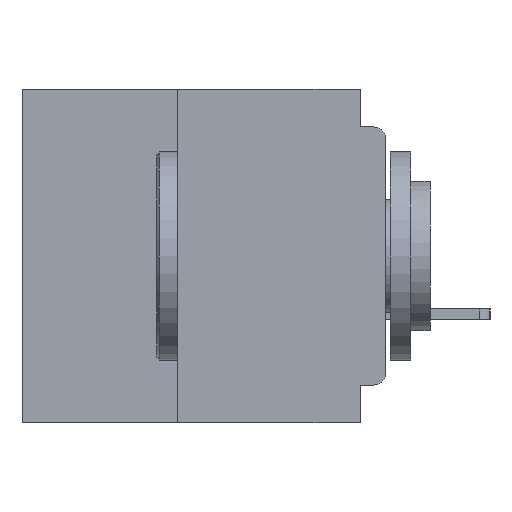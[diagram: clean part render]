
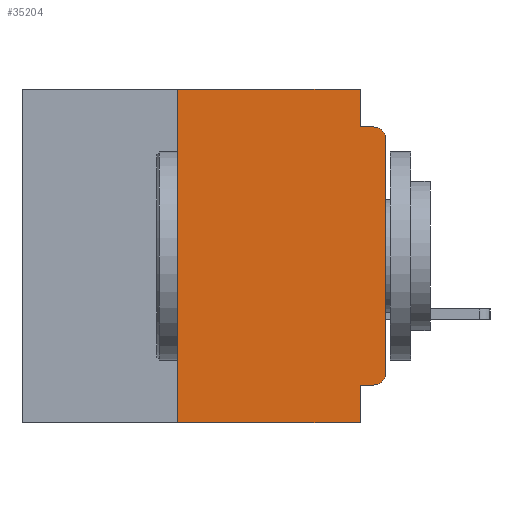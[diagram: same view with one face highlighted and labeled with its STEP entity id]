
A CAD part, left-side view. The second image highlights one B-rep face of the part: STEP entity #35204.
In plain terms, the highlighted planar face has unit normal (-1, 0, 0).
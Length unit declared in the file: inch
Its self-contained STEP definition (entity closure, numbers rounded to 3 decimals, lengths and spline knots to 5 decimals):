
#501 = DIRECTION ( 'NONE',  ( 0., -1., 0. ) ) ;
#698 = CARTESIAN_POINT ( 'NONE',  ( 0., 0.031, 0. ) ) ;
#894 = VECTOR ( 'NONE', #30926, 39.37008 ) ;
#3254 = CARTESIAN_POINT ( 'NONE',  ( 0., 0.25, -0.4 ) ) ;
#5697 = DIRECTION ( 'NONE',  ( 0., 0., -1. ) ) ;
#5958 = DIRECTION ( 'NONE',  ( -1., 0., 0. ) ) ;
#6098 = VERTEX_POINT ( 'NONE', #42554 ) ;
#6409 = CARTESIAN_POINT ( 'NONE',  ( 0., 0.015, -0.06 ) ) ;
#6439 = EDGE_CURVE ( 'NONE', #19492, #18868, #34185, .T. ) ;
#7051 = CARTESIAN_POINT ( 'NONE',  ( 0., 0., 0. ) ) ;
#7656 = LINE ( 'NONE', #34507, #42823 ) ;
#8656 = ORIENTED_EDGE ( 'NONE', *, *, #17409, .T. ) ;
#8794 = FACE_OUTER_BOUND ( 'NONE', #38263, .T. ) ;
#8994 = DIRECTION ( 'NONE',  ( 0., 0., 1. ) ) ;
#9819 = DIRECTION ( 'NONE',  ( 0., 0., -1. ) ) ;
#9920 = CARTESIAN_POINT ( 'NONE',  ( 0., 0., -0.34 ) ) ;
#10199 = EDGE_CURVE ( 'NONE', #22359, #40887, #28156, .T. ) ;
#10862 = LINE ( 'NONE', #26138, #29012 ) ;
#12484 = EDGE_CURVE ( 'NONE', #38335, #40887, #30149, .T. ) ;
#12596 = ORIENTED_EDGE ( 'NONE', *, *, #32562, .T. ) ;
#12644 = AXIS2_PLACEMENT_3D ( 'NONE', #14131, #17571, #41356 ) ;
#13024 = ORIENTED_EDGE ( 'NONE', *, *, #28829, .T. ) ;
#13084 = CARTESIAN_POINT ( 'NONE',  ( 0., 0.031, -0.355 ) ) ;
#14093 = DIRECTION ( 'NONE',  ( 0., 1., 0. ) ) ;
#14131 = CARTESIAN_POINT ( 'NONE',  ( 0., 0.437, 0. ) ) ;
#14196 = ORIENTED_EDGE ( 'NONE', *, *, #10199, .F. ) ;
#14395 = CIRCLE ( 'NONE', #21975, 0.015 ) ;
#16547 = EDGE_CURVE ( 'NONE', #18846, #35949, #22471, .T. ) ;
#17409 = EDGE_CURVE ( 'NONE', #6098, #39542, #14395, .T. ) ;
#17571 = DIRECTION ( 'NONE',  ( 1., 0., 0. ) ) ;
#17613 = CARTESIAN_POINT ( 'NONE',  ( 0., 0.437, -0.4 ) ) ;
#18070 = LINE ( 'NONE', #7051, #894 ) ;
#18543 = ORIENTED_EDGE ( 'NONE', *, *, #16547, .F. ) ;
#18846 = VERTEX_POINT ( 'NONE', #21223 ) ;
#18868 = VERTEX_POINT ( 'NONE', #698 ) ;
#18967 = DIRECTION ( 'NONE',  ( 0., 0., -1. ) ) ;
#19480 = ORIENTED_EDGE ( 'NONE', *, *, #12484, .T. ) ;
#19492 = VERTEX_POINT ( 'NONE', #21315 ) ;
#20513 = DIRECTION ( 'NONE',  ( 0., -1., 0. ) ) ;
#21223 = CARTESIAN_POINT ( 'NONE',  ( 0., 0.031, -0.045 ) ) ;
#21315 = CARTESIAN_POINT ( 'NONE',  ( 0., 0.25, 0. ) ) ;
#21417 = VECTOR ( 'NONE', #29590, 39.37008 ) ;
#21463 = AXIS2_PLACEMENT_3D ( 'NONE', #6409, #30259, #9819 ) ;
#21652 = EDGE_CURVE ( 'NONE', #38335, #19492, #30915, .T. ) ;
#21975 = AXIS2_PLACEMENT_3D ( 'NONE', #26390, #5958, #29835 ) ;
#22359 = VERTEX_POINT ( 'NONE', #13084 ) ;
#22405 = CARTESIAN_POINT ( 'NONE',  ( 0., 0.015, -0.045 ) ) ;
#22471 = LINE ( 'NONE', #32877, #21417 ) ;
#23923 = EDGE_CURVE ( 'NONE', #18868, #18846, #10862, .T. ) ;
#25971 = CARTESIAN_POINT ( 'NONE',  ( 0., 0.25, -0.4 ) ) ;
#26138 = CARTESIAN_POINT ( 'NONE',  ( 0., 0.031, 0. ) ) ;
#26390 = CARTESIAN_POINT ( 'NONE',  ( 0., 0.015, -0.34 ) ) ;
#27092 = VECTOR ( 'NONE', #18967, 39.37008 ) ;
#27287 = ORIENTED_EDGE ( 'NONE', *, *, #6439, .F. ) ;
#27679 = PLANE ( 'NONE',  #12644 ) ;
#28156 = LINE ( 'NONE', #39337, #27092 ) ;
#28829 = EDGE_CURVE ( 'NONE', #30629, #35949, #37508, .T. ) ;
#29012 = VECTOR ( 'NONE', #5697, 39.37008 ) ;
#29590 = DIRECTION ( 'NONE',  ( 0., -1., 0. ) ) ;
#29835 = DIRECTION ( 'NONE',  ( 0., 0., -1. ) ) ;
#30149 = LINE ( 'NONE', #17613, #38116 ) ;
#30259 = DIRECTION ( 'NONE',  ( -1., 0., 0. ) ) ;
#30629 = VERTEX_POINT ( 'NONE', #32942 ) ;
#30915 = LINE ( 'NONE', #25971, #38854 ) ;
#30926 = DIRECTION ( 'NONE',  ( 0., 0., 1. ) ) ;
#32562 = EDGE_CURVE ( 'NONE', #39542, #30629, #18070, .T. ) ;
#32877 = CARTESIAN_POINT ( 'NONE',  ( 0., 0., -0.045 ) ) ;
#32942 = CARTESIAN_POINT ( 'NONE',  ( 0., 0., -0.06 ) ) ;
#34185 = LINE ( 'NONE', #44289, #41064 ) ;
#34507 = CARTESIAN_POINT ( 'NONE',  ( 0., 0., -0.355 ) ) ;
#35204 = ADVANCED_FACE ( 'NONE', ( #8794 ), #27679, .F. ) ;
#35669 = EDGE_CURVE ( 'NONE', #6098, #22359, #7656, .T. ) ;
#35949 = VERTEX_POINT ( 'NONE', #22405 ) ;
#37508 = CIRCLE ( 'NONE', #21463, 0.015 ) ;
#38116 = VECTOR ( 'NONE', #501, 39.37008 ) ;
#38263 = EDGE_LOOP ( 'NONE', ( #12596, #13024, #18543, #40934, #27287, #40049, #19480, #14196, #43642, #8656 ) ) ;
#38335 = VERTEX_POINT ( 'NONE', #3254 ) ;
#38854 = VECTOR ( 'NONE', #8994, 39.37008 ) ;
#39337 = CARTESIAN_POINT ( 'NONE',  ( 0., 0.031, -0.4 ) ) ;
#39542 = VERTEX_POINT ( 'NONE', #9920 ) ;
#40049 = ORIENTED_EDGE ( 'NONE', *, *, #21652, .F. ) ;
#40887 = VERTEX_POINT ( 'NONE', #43152 ) ;
#40934 = ORIENTED_EDGE ( 'NONE', *, *, #23923, .F. ) ;
#41064 = VECTOR ( 'NONE', #20513, 39.37008 ) ;
#41356 = DIRECTION ( 'NONE',  ( 0., 0., -1. ) ) ;
#42554 = CARTESIAN_POINT ( 'NONE',  ( 0., 0.015, -0.355 ) ) ;
#42823 = VECTOR ( 'NONE', #14093, 39.37008 ) ;
#43152 = CARTESIAN_POINT ( 'NONE',  ( 0., 0.031, -0.4 ) ) ;
#43642 = ORIENTED_EDGE ( 'NONE', *, *, #35669, .F. ) ;
#44289 = CARTESIAN_POINT ( 'NONE',  ( 0., 0.437, 0. ) ) ;
